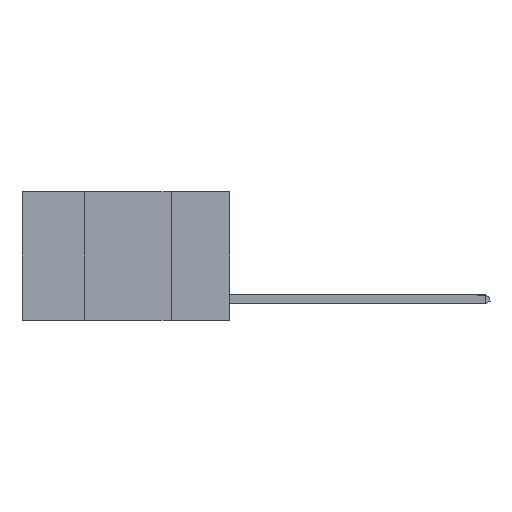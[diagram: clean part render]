
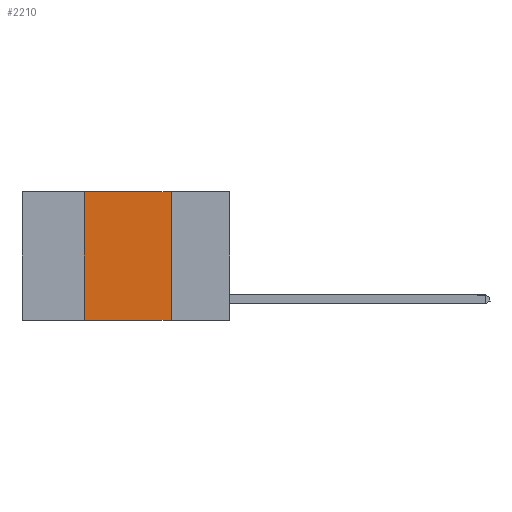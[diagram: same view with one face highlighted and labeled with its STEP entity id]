
A CAD part, left-side view. The second image highlights one B-rep face of the part: STEP entity #2210.
In plain terms, the highlighted planar face has unit normal (-1, 0, 0).
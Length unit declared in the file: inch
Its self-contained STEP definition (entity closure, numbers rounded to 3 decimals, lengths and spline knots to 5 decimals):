
#571 = CARTESIAN_POINT ( 'NONE',  ( 0., 0.17, -0.37 ) ) ;
#636 = CARTESIAN_POINT ( 'NONE',  ( 0., 0.6, 0. ) ) ;
#704 = CARTESIAN_POINT ( 'NONE',  ( 0., 0.17, 0. ) ) ;
#1159 = EDGE_CURVE ( 'NONE', #1617, #10346, #1374, .T. ) ;
#1374 = LINE ( 'NONE', #3568, #7565 ) ;
#1617 = VERTEX_POINT ( 'NONE', #8336 ) ;
#2026 = DIRECTION ( 'NONE',  ( 0., 0., -1. ) ) ;
#2210 = ADVANCED_FACE ( 'NONE', ( #4463 ), #9874, .F. ) ;
#2360 = DIRECTION ( 'NONE',  ( 0., 0., -1. ) ) ;
#2570 = VECTOR ( 'NONE', #8185, 39.37008 ) ;
#2651 = VERTEX_POINT ( 'NONE', #704 ) ;
#2704 = DIRECTION ( 'NONE',  ( 0., 0., 1. ) ) ;
#2975 = EDGE_LOOP ( 'NONE', ( #8700, #7078, #10433, #10578 ) ) ;
#3206 = CARTESIAN_POINT ( 'NONE',  ( 0., 0.6, -0.37 ) ) ;
#3568 = CARTESIAN_POINT ( 'NONE',  ( 0., 0.42, 0. ) ) ;
#4038 = VECTOR ( 'NONE', #2026, 39.37008 ) ;
#4463 = FACE_OUTER_BOUND ( 'NONE', #2975, .T. ) ;
#4843 = LINE ( 'NONE', #3206, #2570 ) ;
#5576 = AXIS2_PLACEMENT_3D ( 'NONE', #636, #7401, #2360 ) ;
#5767 = CARTESIAN_POINT ( 'NONE',  ( 0., 0.6, 0. ) ) ;
#6968 = EDGE_CURVE ( 'NONE', #1617, #8131, #4843, .T. ) ;
#7078 = ORIENTED_EDGE ( 'NONE', *, *, #10745, .F. ) ;
#7401 = DIRECTION ( 'NONE',  ( 1., 0., 0. ) ) ;
#7565 = VECTOR ( 'NONE', #2704, 39.37008 ) ;
#7911 = CARTESIAN_POINT ( 'NONE',  ( 0., 0.17, 0. ) ) ;
#7935 = EDGE_CURVE ( 'NONE', #2651, #8131, #10372, .T. ) ;
#8131 = VERTEX_POINT ( 'NONE', #571 ) ;
#8185 = DIRECTION ( 'NONE',  ( 0., -1., 0. ) ) ;
#8336 = CARTESIAN_POINT ( 'NONE',  ( 0., 0.42, -0.37 ) ) ;
#8495 = VECTOR ( 'NONE', #9091, 39.37008 ) ;
#8700 = ORIENTED_EDGE ( 'NONE', *, *, #7935, .F. ) ;
#9091 = DIRECTION ( 'NONE',  ( 0., -1., 0. ) ) ;
#9874 = PLANE ( 'NONE',  #5576 ) ;
#10256 = CARTESIAN_POINT ( 'NONE',  ( 0., 0.42, 0. ) ) ;
#10346 = VERTEX_POINT ( 'NONE', #10256 ) ;
#10372 = LINE ( 'NONE', #7911, #4038 ) ;
#10433 = ORIENTED_EDGE ( 'NONE', *, *, #1159, .F. ) ;
#10578 = ORIENTED_EDGE ( 'NONE', *, *, #6968, .T. ) ;
#10692 = LINE ( 'NONE', #5767, #8495 ) ;
#10745 = EDGE_CURVE ( 'NONE', #10346, #2651, #10692, .T. ) ;
